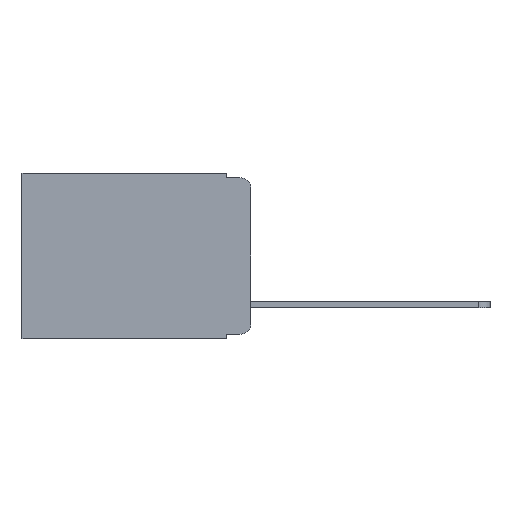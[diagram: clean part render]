
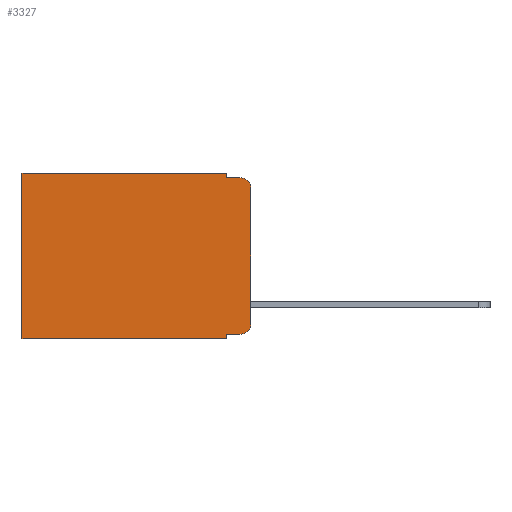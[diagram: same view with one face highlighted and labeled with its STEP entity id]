
A CAD part, left-side view. The second image highlights one B-rep face of the part: STEP entity #3327.
In plain terms, the highlighted planar face has unit normal (-1, 0, 0).
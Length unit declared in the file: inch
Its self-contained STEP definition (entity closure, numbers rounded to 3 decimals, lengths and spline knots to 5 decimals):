
#10 = DIRECTION ( 'NONE',  ( 0., 0., -1. ) ) ;
#745 = LINE ( 'NONE', #1937, #3941 ) ;
#765 = DIRECTION ( 'NONE',  ( 0., -1., 0. ) ) ;
#975 = PLANE ( 'NONE',  #7127 ) ;
#987 = VERTEX_POINT ( 'NONE', #1210 ) ;
#1089 = DIRECTION ( 'NONE',  ( 0., 0., -1. ) ) ;
#1210 = CARTESIAN_POINT ( 'NONE',  ( 0.298, 0.051, -0.333 ) ) ;
#1238 = CARTESIAN_POINT ( 'NONE',  ( 0.298, 0.02, -0.333 ) ) ;
#1482 = CARTESIAN_POINT ( 'NONE',  ( 0.298, 0.473, 0. ) ) ;
#1689 = CARTESIAN_POINT ( 'NONE',  ( 0.298, 0., -0.03 ) ) ;
#1937 = CARTESIAN_POINT ( 'NONE',  ( 0.298, 0.051, -0.333 ) ) ;
#2408 = LINE ( 'NONE', #16377, #14882 ) ;
#3234 = VERTEX_POINT ( 'NONE', #4160 ) ;
#3288 = CARTESIAN_POINT ( 'NONE',  ( 0.298, 0.02, -0.03 ) ) ;
#3327 = ADVANCED_FACE ( 'NONE', ( #13577 ), #975, .F. ) ;
#3389 = VERTEX_POINT ( 'NONE', #1482 ) ;
#3534 = CIRCLE ( 'NONE', #7514, 0.02 ) ;
#3732 = ORIENTED_EDGE ( 'NONE', *, *, #10397, .F. ) ;
#3750 = ORIENTED_EDGE ( 'NONE', *, *, #5690, .F. ) ;
#3941 = VECTOR ( 'NONE', #765, 39.37008 ) ;
#3997 = LINE ( 'NONE', #16637, #9000 ) ;
#4133 = CARTESIAN_POINT ( 'NONE',  ( 0.298, 0.02, -0.01 ) ) ;
#4160 = CARTESIAN_POINT ( 'NONE',  ( 0.298, 0.051, -0.343 ) ) ;
#4269 = ORIENTED_EDGE ( 'NONE', *, *, #11724, .T. ) ;
#4289 = DIRECTION ( 'NONE',  ( 0., 1., 0. ) ) ;
#4642 = AXIS2_PLACEMENT_3D ( 'NONE', #8869, #7513, #1089 ) ;
#4682 = DIRECTION ( 'NONE',  ( -1., 0., 0. ) ) ;
#4694 = VECTOR ( 'NONE', #10, 39.37008 ) ;
#4905 = VECTOR ( 'NONE', #14487, 39.37008 ) ;
#5520 = CARTESIAN_POINT ( 'NONE',  ( 0.298, 0.051, 0. ) ) ;
#5690 = EDGE_CURVE ( 'NONE', #3234, #11415, #2408, .T. ) ;
#5931 = VERTEX_POINT ( 'NONE', #4133 ) ;
#6315 = ORIENTED_EDGE ( 'NONE', *, *, #14371, .T. ) ;
#6320 = DIRECTION ( 'NONE',  ( 0., -1., 0. ) ) ;
#6695 = LINE ( 'NONE', #15890, #4905 ) ;
#6773 = ORIENTED_EDGE ( 'NONE', *, *, #12030, .F. ) ;
#6795 = VERTEX_POINT ( 'NONE', #1689 ) ;
#7016 = CARTESIAN_POINT ( 'NONE',  ( 0.298, 0.051, -0.01 ) ) ;
#7127 = AXIS2_PLACEMENT_3D ( 'NONE', #7400, #8695, #10088 ) ;
#7205 = VECTOR ( 'NONE', #11725, 39.37008 ) ;
#7400 = CARTESIAN_POINT ( 'NONE',  ( 0.298, 0., 0. ) ) ;
#7513 = DIRECTION ( 'NONE',  ( -1., 0., 0. ) ) ;
#7514 = AXIS2_PLACEMENT_3D ( 'NONE', #3288, #4682, #12238 ) ;
#7865 = CARTESIAN_POINT ( 'NONE',  ( 0.298, 0.051, 0. ) ) ;
#8077 = VERTEX_POINT ( 'NONE', #8847 ) ;
#8158 = VECTOR ( 'NONE', #4289, 39.37008 ) ;
#8612 = DIRECTION ( 'NONE',  ( 0., 1., 0. ) ) ;
#8695 = DIRECTION ( 'NONE',  ( 1., 0., 0. ) ) ;
#8763 = DIRECTION ( 'NONE',  ( 0., 0., -1. ) ) ;
#8805 = EDGE_CURVE ( 'NONE', #987, #3234, #10480, .T. ) ;
#8847 = CARTESIAN_POINT ( 'NONE',  ( 0.298, 0., -0.313 ) ) ;
#8869 = CARTESIAN_POINT ( 'NONE',  ( 0.298, 0.02, -0.313 ) ) ;
#9000 = VECTOR ( 'NONE', #6320, 39.37008 ) ;
#9224 = CARTESIAN_POINT ( 'NONE',  ( 0.298, 0., 0. ) ) ;
#10088 = DIRECTION ( 'NONE',  ( 0., 0., -1. ) ) ;
#10178 = CIRCLE ( 'NONE', #4642, 0.02 ) ;
#10343 = LINE ( 'NONE', #15472, #4694 ) ;
#10356 = ORIENTED_EDGE ( 'NONE', *, *, #12709, .T. ) ;
#10373 = ORIENTED_EDGE ( 'NONE', *, *, #12085, .T. ) ;
#10397 = EDGE_CURVE ( 'NONE', #14646, #5931, #3997, .T. ) ;
#10428 = VERTEX_POINT ( 'NONE', #1238 ) ;
#10480 = LINE ( 'NONE', #7865, #7205 ) ;
#10601 = CARTESIAN_POINT ( 'NONE',  ( 0.298, 0.473, -0.343 ) ) ;
#10845 = ORIENTED_EDGE ( 'NONE', *, *, #11752, .T. ) ;
#11415 = VERTEX_POINT ( 'NONE', #10601 ) ;
#11724 = EDGE_CURVE ( 'NONE', #987, #10428, #745, .T. ) ;
#11725 = DIRECTION ( 'NONE',  ( 0., 0., -1. ) ) ;
#11752 = EDGE_CURVE ( 'NONE', #6795, #5931, #3534, .T. ) ;
#12030 = EDGE_CURVE ( 'NONE', #12745, #14646, #12776, .T. ) ;
#12085 = EDGE_CURVE ( 'NONE', #10428, #8077, #10178, .T. ) ;
#12202 = VECTOR ( 'NONE', #8763, 39.37008 ) ;
#12238 = DIRECTION ( 'NONE',  ( 0., 0., -1. ) ) ;
#12709 = EDGE_CURVE ( 'NONE', #12745, #3389, #14215, .T. ) ;
#12745 = VERTEX_POINT ( 'NONE', #5520 ) ;
#12776 = LINE ( 'NONE', #16490, #12202 ) ;
#13577 = FACE_OUTER_BOUND ( 'NONE', #16015, .T. ) ;
#13927 = EDGE_CURVE ( 'NONE', #6795, #8077, #6695, .T. ) ;
#14215 = LINE ( 'NONE', #9224, #8158 ) ;
#14371 = EDGE_CURVE ( 'NONE', #3389, #11415, #10343, .T. ) ;
#14487 = DIRECTION ( 'NONE',  ( 0., 0., -1. ) ) ;
#14521 = ORIENTED_EDGE ( 'NONE', *, *, #8805, .F. ) ;
#14585 = ORIENTED_EDGE ( 'NONE', *, *, #13927, .F. ) ;
#14646 = VERTEX_POINT ( 'NONE', #7016 ) ;
#14882 = VECTOR ( 'NONE', #8612, 39.37008 ) ;
#15472 = CARTESIAN_POINT ( 'NONE',  ( 0.298, 0.473, 0. ) ) ;
#15890 = CARTESIAN_POINT ( 'NONE',  ( 0.298, 0., 0. ) ) ;
#16015 = EDGE_LOOP ( 'NONE', ( #14585, #10845, #3732, #6773, #10356, #6315, #3750, #14521, #4269, #10373 ) ) ;
#16377 = CARTESIAN_POINT ( 'NONE',  ( 0.298, 0., -0.343 ) ) ;
#16490 = CARTESIAN_POINT ( 'NONE',  ( 0.298, 0.051, 0. ) ) ;
#16637 = CARTESIAN_POINT ( 'NONE',  ( 0.298, 0.051, -0.01 ) ) ;
